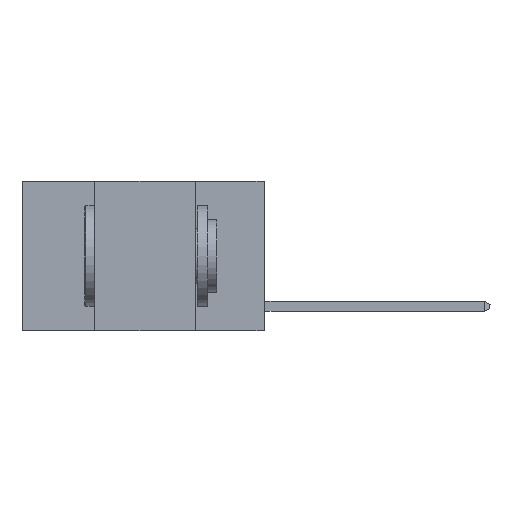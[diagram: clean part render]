
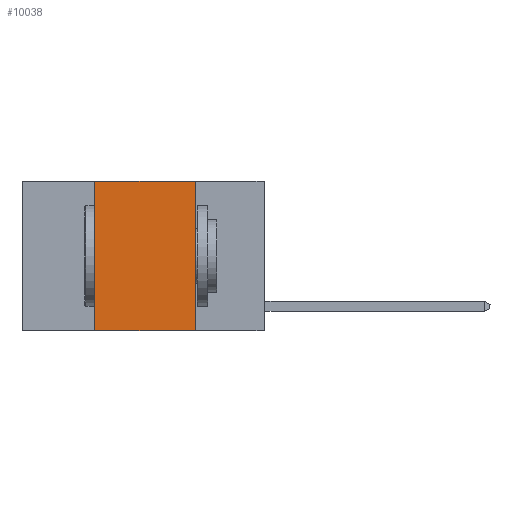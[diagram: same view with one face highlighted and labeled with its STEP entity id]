
A CAD part, left-side view. The second image highlights one B-rep face of the part: STEP entity #10038.
In plain terms, the highlighted planar face has unit normal (-1, 0, 0).
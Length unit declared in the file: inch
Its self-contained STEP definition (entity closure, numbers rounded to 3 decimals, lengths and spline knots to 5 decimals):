
#461 = ORIENTED_EDGE ( 'NONE', *, *, #6385, .F. ) ;
#1121 = VERTEX_POINT ( 'NONE', #21602 ) ;
#1537 = ORIENTED_EDGE ( 'NONE', *, *, #13181, .F. ) ;
#2403 = PLANE ( 'NONE',  #21907 ) ;
#2606 = FACE_OUTER_BOUND ( 'NONE', #4139, .T. ) ;
#3534 = CARTESIAN_POINT ( 'NONE',  ( 0., 0.6, -0.37 ) ) ;
#4139 = EDGE_LOOP ( 'NONE', ( #18407, #1537, #461, #12180 ) ) ;
#5303 = DIRECTION ( 'NONE',  ( 0., -1., 0. ) ) ;
#5759 = CARTESIAN_POINT ( 'NONE',  ( 0., 0.17, -0.37 ) ) ;
#5941 = CARTESIAN_POINT ( 'NONE',  ( 0., 0.6, 0. ) ) ;
#6385 = EDGE_CURVE ( 'NONE', #1121, #14863, #19715, .T. ) ;
#6634 = VECTOR ( 'NONE', #10988, 39.37008 ) ;
#7166 = LINE ( 'NONE', #17880, #6634 ) ;
#7715 = DIRECTION ( 'NONE',  ( 0., 0., -1. ) ) ;
#9981 = VECTOR ( 'NONE', #15886, 39.37008 ) ;
#10038 = ADVANCED_FACE ( 'NONE', ( #2606 ), #2403, .F. ) ;
#10056 = CARTESIAN_POINT ( 'NONE',  ( 0., 0.42, 0. ) ) ;
#10642 = CARTESIAN_POINT ( 'NONE',  ( 0., 0.42, 0. ) ) ;
#10988 = DIRECTION ( 'NONE',  ( 0., 0., -1. ) ) ;
#12180 = ORIENTED_EDGE ( 'NONE', *, *, #16155, .T. ) ;
#13181 = EDGE_CURVE ( 'NONE', #14863, #20352, #16939, .T. ) ;
#14364 = CARTESIAN_POINT ( 'NONE',  ( 0., 0.17, 0. ) ) ;
#14863 = VERTEX_POINT ( 'NONE', #10056 ) ;
#15739 = CARTESIAN_POINT ( 'NONE',  ( 0., 0.6, 0. ) ) ;
#15886 = DIRECTION ( 'NONE',  ( 0., 0., 1. ) ) ;
#16155 = EDGE_CURVE ( 'NONE', #1121, #21642, #21202, .T. ) ;
#16939 = LINE ( 'NONE', #15739, #20953 ) ;
#17460 = DIRECTION ( 'NONE',  ( 0., -1., 0. ) ) ;
#17880 = CARTESIAN_POINT ( 'NONE',  ( 0., 0.17, 0. ) ) ;
#18122 = DIRECTION ( 'NONE',  ( 1., 0., 0. ) ) ;
#18407 = ORIENTED_EDGE ( 'NONE', *, *, #21604, .F. ) ;
#19715 = LINE ( 'NONE', #10642, #9981 ) ;
#20352 = VERTEX_POINT ( 'NONE', #14364 ) ;
#20668 = VECTOR ( 'NONE', #5303, 39.37008 ) ;
#20953 = VECTOR ( 'NONE', #17460, 39.37008 ) ;
#21202 = LINE ( 'NONE', #3534, #20668 ) ;
#21602 = CARTESIAN_POINT ( 'NONE',  ( 0., 0.42, -0.37 ) ) ;
#21604 = EDGE_CURVE ( 'NONE', #20352, #21642, #7166, .T. ) ;
#21642 = VERTEX_POINT ( 'NONE', #5759 ) ;
#21907 = AXIS2_PLACEMENT_3D ( 'NONE', #5941, #18122, #7715 ) ;
